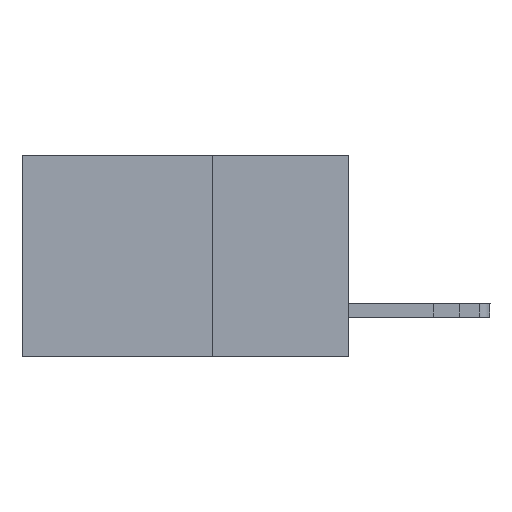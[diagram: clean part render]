
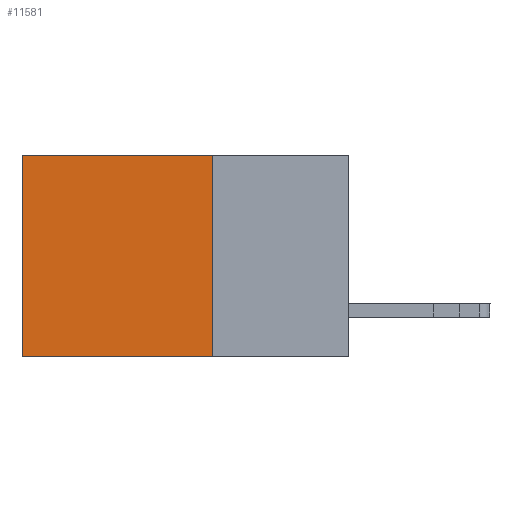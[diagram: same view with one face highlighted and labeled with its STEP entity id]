
A CAD part, left-side view. The second image highlights one B-rep face of the part: STEP entity #11581.
In plain terms, the highlighted planar face has unit normal (-1, 0, 0).
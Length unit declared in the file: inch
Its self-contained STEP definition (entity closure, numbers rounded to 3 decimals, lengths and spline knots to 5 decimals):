
#130 = ORIENTED_EDGE ( 'NONE', *, *, #5503, .F. ) ;
#219 = VECTOR ( 'NONE', #5632, 39.37008 ) ;
#359 = DIRECTION ( 'NONE',  ( 0., 0., -1. ) ) ;
#552 = LINE ( 'NONE', #5433, #219 ) ;
#1309 = VECTOR ( 'NONE', #8933, 39.37008 ) ;
#2155 = CARTESIAN_POINT ( 'NONE',  ( 0.2615, 0.25, -0.37 ) ) ;
#2692 = DIRECTION ( 'NONE',  ( 1., 0., 0. ) ) ;
#2771 = CARTESIAN_POINT ( 'NONE',  ( 0.2615, 0.6, 0. ) ) ;
#3442 = VERTEX_POINT ( 'NONE', #4594 ) ;
#3945 = ORIENTED_EDGE ( 'NONE', *, *, #9117, .F. ) ;
#3974 = LINE ( 'NONE', #6038, #7931 ) ;
#4594 = CARTESIAN_POINT ( 'NONE',  ( 0.2615, 0.25, 0. ) ) ;
#5433 = CARTESIAN_POINT ( 'NONE',  ( 0.2615, 0.25, 0. ) ) ;
#5503 = EDGE_CURVE ( 'NONE', #3442, #6738, #9996, .T. ) ;
#5521 = CARTESIAN_POINT ( 'NONE',  ( 0.2615, 0.6, -0.37 ) ) ;
#5584 = CARTESIAN_POINT ( 'NONE',  ( 0.2615, 0.6, -0.37 ) ) ;
#5632 = DIRECTION ( 'NONE',  ( 0., 1., 0. ) ) ;
#5702 = DIRECTION ( 'NONE',  ( 0., 0., -1. ) ) ;
#6038 = CARTESIAN_POINT ( 'NONE',  ( 0.2615, 0.25, -0.37 ) ) ;
#6738 = VERTEX_POINT ( 'NONE', #2155 ) ;
#7931 = VECTOR ( 'NONE', #10943, 39.37008 ) ;
#8835 = VERTEX_POINT ( 'NONE', #2771 ) ;
#8933 = DIRECTION ( 'NONE',  ( 0., 0., -1. ) ) ;
#9117 = EDGE_CURVE ( 'NONE', #6738, #13232, #3974, .T. ) ;
#9272 = ORIENTED_EDGE ( 'NONE', *, *, #10632, .T. ) ;
#9461 = EDGE_LOOP ( 'NONE', ( #10152, #3945, #130, #9272 ) ) ;
#9606 = CARTESIAN_POINT ( 'NONE',  ( 0.2615, 0.25, -0.37 ) ) ;
#9768 = VECTOR ( 'NONE', #5702, 39.37008 ) ;
#9793 = CARTESIAN_POINT ( 'NONE',  ( 0.2615, 0.25, -0.37 ) ) ;
#9996 = LINE ( 'NONE', #9793, #9768 ) ;
#10152 = ORIENTED_EDGE ( 'NONE', *, *, #13251, .T. ) ;
#10632 = EDGE_CURVE ( 'NONE', #3442, #8835, #552, .T. ) ;
#10943 = DIRECTION ( 'NONE',  ( 0., 1., 0. ) ) ;
#11004 = LINE ( 'NONE', #5584, #1309 ) ;
#11581 = ADVANCED_FACE ( 'NONE', ( #12828 ), #12887, .F. ) ;
#12483 = AXIS2_PLACEMENT_3D ( 'NONE', #9606, #2692, #359 ) ;
#12828 = FACE_OUTER_BOUND ( 'NONE', #9461, .T. ) ;
#12887 = PLANE ( 'NONE',  #12483 ) ;
#13232 = VERTEX_POINT ( 'NONE', #5521 ) ;
#13251 = EDGE_CURVE ( 'NONE', #8835, #13232, #11004, .T. ) ;
